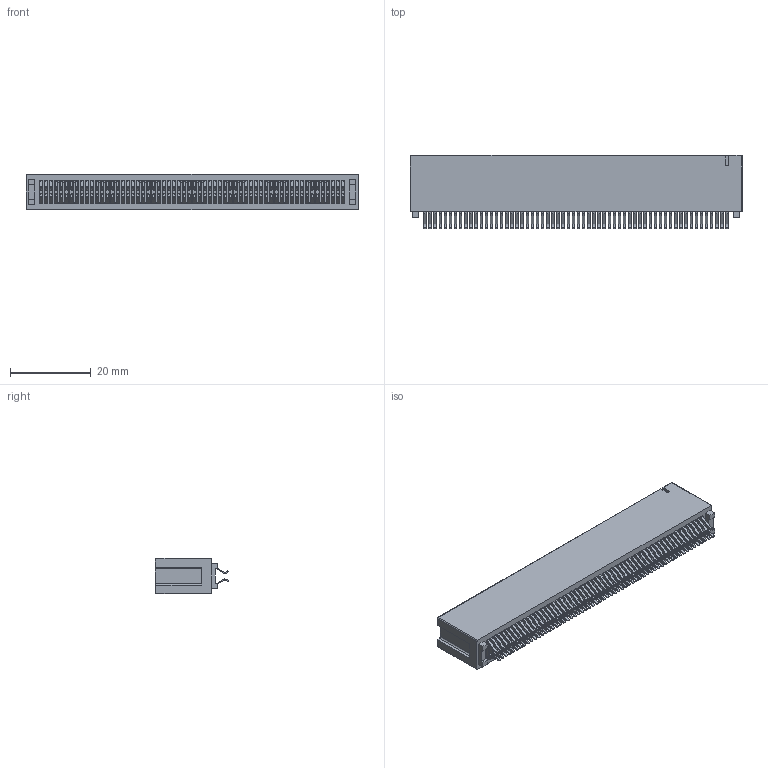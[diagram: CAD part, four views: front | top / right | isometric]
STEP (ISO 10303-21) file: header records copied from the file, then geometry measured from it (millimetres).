
FILE_DESCRIPTION (( 'STEP AP203' ), '1' );
FILE_NAME ('302-120-256-201.STEP', '2024-04-06T14:37:25', ( '' ), ( '' ), 'SwSTEP 2.0', 'SolidWorks 2023', '' );
FILE_SCHEMA (( 'CONFIG_CONTROL_DESIGN' ));
Length unit declared in the file: millimetre
Products named in the file (3): 302-120-256-201; Contact_302-290-X56; HSG_Vertical HSG
Assembly tree (121 placements, depth 2):
  302-120-256-201
    HSG_Vertical HSG
    Contact_302-290-X56  x120
Bounding box: 82.3 x 18.3 x 8.88 mm (x, y, z)
Volume: 6274.7 mm3; surface area: 18134.8 mm2
Topology: 121 solids, 121 shells, 5766 faces, 17208 edges, 11384 vertices
Faces by surface type: plane 3829, cylinder 1933, sphere 4
Entity records: 44895 total; most frequent: ORIENTED_EDGE 7752, CARTESIAN_POINT 7604, DIRECTION 6186, EDGE_CURVE 3876, VECTOR 3818, LINE 3818, VERTEX_POINT 2578, EDGE_LOOP 1190
